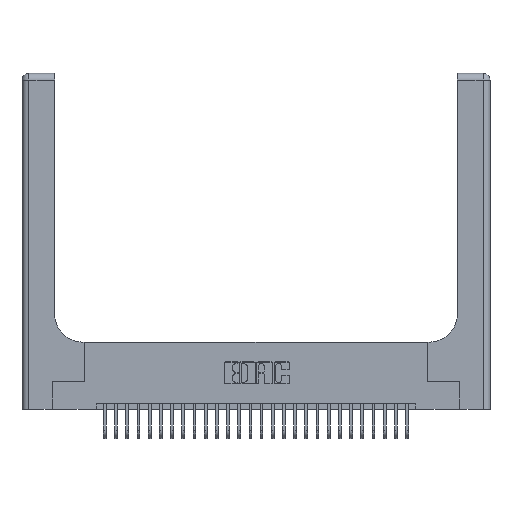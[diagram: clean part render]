
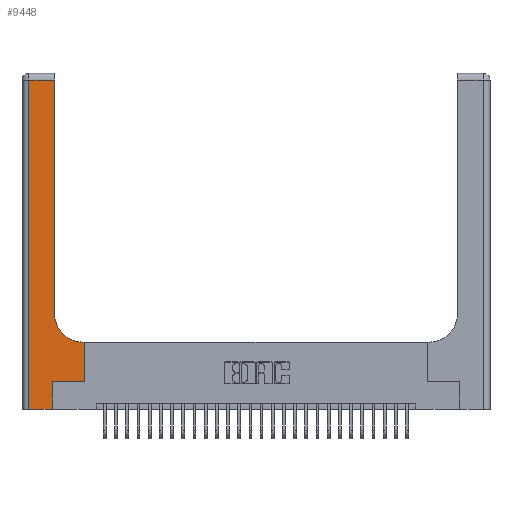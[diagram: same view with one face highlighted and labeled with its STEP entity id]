
A CAD part, top view. The second image highlights one B-rep face of the part: STEP entity #9448.
In plain terms, the highlighted planar face has unit normal (0, 0, 1).
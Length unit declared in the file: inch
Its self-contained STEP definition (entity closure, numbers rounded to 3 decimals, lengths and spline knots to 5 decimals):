
#297 = CARTESIAN_POINT ( 'NONE',  ( 0., 3., 0.37 ) ) ;
#1037 = CARTESIAN_POINT ( 'NONE',  ( 0.269, 0.25, 0.37 ) ) ;
#1071 = EDGE_CURVE ( 'NONE', #6506, #24500, #28959, .T. ) ;
#1226 = VECTOR ( 'NONE', #18215, 39.37008 ) ;
#2279 = ORIENTED_EDGE ( 'NONE', *, *, #6819, .T. ) ;
#3363 = DIRECTION ( 'NONE',  ( 0., -1., 0. ) ) ;
#3562 = EDGE_CURVE ( 'NONE', #7174, #15607, #13277, .T. ) ;
#3978 = EDGE_CURVE ( 'NONE', #15607, #24479, #28033, .T. ) ;
#5004 = PLANE ( 'NONE',  #11154 ) ;
#5107 = DIRECTION ( 'NONE',  ( -1., 0., 0. ) ) ;
#5175 = EDGE_CURVE ( 'NONE', #20872, #12508, #20188, .T. ) ;
#5329 = CARTESIAN_POINT ( 'NONE',  ( 0.5585, 0.6, 0.37 ) ) ;
#5599 = EDGE_CURVE ( 'NONE', #24479, #21643, #9063, .T. ) ;
#6296 = ORIENTED_EDGE ( 'NONE', *, *, #5175, .T. ) ;
#6438 = CARTESIAN_POINT ( 'NONE',  ( 0.06, 0., 0.37 ) ) ;
#6506 = VERTEX_POINT ( 'NONE', #30157 ) ;
#6819 = EDGE_CURVE ( 'NONE', #18335, #6506, #7108, .T. ) ;
#6947 = DIRECTION ( 'NONE',  ( 0., 1., 0. ) ) ;
#7108 = LINE ( 'NONE', #7600, #19004 ) ;
#7174 = VERTEX_POINT ( 'NONE', #6438 ) ;
#7600 = CARTESIAN_POINT ( 'NONE',  ( 0.2915, 0.6, 0.37 ) ) ;
#7916 = CARTESIAN_POINT ( 'NONE',  ( 0.2915, 0.85, 0.37 ) ) ;
#8496 = DIRECTION ( 'NONE',  ( 0., 0., -1. ) ) ;
#8878 = LINE ( 'NONE', #11604, #13674 ) ;
#8983 = LINE ( 'NONE', #17615, #21556 ) ;
#9063 = LINE ( 'NONE', #1037, #14609 ) ;
#9194 = VECTOR ( 'NONE', #16096, 39.37008 ) ;
#9448 = ADVANCED_FACE ( 'NONE', ( #24695 ), #5004, .F. ) ;
#10144 = DIRECTION ( 'NONE',  ( 0., 1., 0. ) ) ;
#10786 = ORIENTED_EDGE ( 'NONE', *, *, #28792, .T. ) ;
#11154 = AXIS2_PLACEMENT_3D ( 'NONE', #297, #19344, #5107 ) ;
#11604 = CARTESIAN_POINT ( 'NONE',  ( 0.2915, 3., 0.37 ) ) ;
#11655 = ORIENTED_EDGE ( 'NONE', *, *, #3978, .T. ) ;
#12508 = VERTEX_POINT ( 'NONE', #23676 ) ;
#12780 = EDGE_CURVE ( 'NONE', #12508, #7174, #8983, .T. ) ;
#13107 = ORIENTED_EDGE ( 'NONE', *, *, #3562, .T. ) ;
#13277 = LINE ( 'NONE', #28307, #19588 ) ;
#13674 = VECTOR ( 'NONE', #6947, 39.37008 ) ;
#13714 = CARTESIAN_POINT ( 'NONE',  ( 0.269, 0., 0.37 ) ) ;
#14431 = ORIENTED_EDGE ( 'NONE', *, *, #12780, .T. ) ;
#14609 = VECTOR ( 'NONE', #27053, 39.37008 ) ;
#14793 = AXIS2_PLACEMENT_3D ( 'NONE', #22649, #8496, #25015 ) ;
#15607 = VERTEX_POINT ( 'NONE', #27298 ) ;
#16096 = DIRECTION ( 'NONE',  ( 0., 1., 0. ) ) ;
#16605 = LINE ( 'NONE', #17167, #22137 ) ;
#17079 = ORIENTED_EDGE ( 'NONE', *, *, #1071, .T. ) ;
#17167 = CARTESIAN_POINT ( 'NONE',  ( 0.5585, 0.25, 0.37 ) ) ;
#17615 = CARTESIAN_POINT ( 'NONE',  ( 0.06, 3., 0.37 ) ) ;
#18215 = DIRECTION ( 'NONE',  ( -1., 0., 0. ) ) ;
#18334 = EDGE_CURVE ( 'NONE', #21643, #18335, #16605, .T. ) ;
#18335 = VERTEX_POINT ( 'NONE', #5329 ) ;
#19004 = VECTOR ( 'NONE', #28909, 39.37008 ) ;
#19344 = DIRECTION ( 'NONE',  ( 0., 0., -1. ) ) ;
#19588 = VECTOR ( 'NONE', #30686, 39.37008 ) ;
#19724 = CARTESIAN_POINT ( 'NONE',  ( 0.269, 0.25, 0.37 ) ) ;
#20188 = LINE ( 'NONE', #29944, #1226 ) ;
#20872 = VERTEX_POINT ( 'NONE', #29404 ) ;
#21476 = EDGE_LOOP ( 'NONE', ( #10786, #6296, #14431, #13107, #11655, #26760, #26188, #2279, #17079 ) ) ;
#21556 = VECTOR ( 'NONE', #3363, 39.37008 ) ;
#21643 = VERTEX_POINT ( 'NONE', #27486 ) ;
#22137 = VECTOR ( 'NONE', #10144, 39.37008 ) ;
#22649 = CARTESIAN_POINT ( 'NONE',  ( 0.5415, 0.85, 0.37 ) ) ;
#23676 = CARTESIAN_POINT ( 'NONE',  ( 0.06, 2.94, 0.37 ) ) ;
#24479 = VERTEX_POINT ( 'NONE', #19724 ) ;
#24500 = VERTEX_POINT ( 'NONE', #7916 ) ;
#24695 = FACE_OUTER_BOUND ( 'NONE', #21476, .T. ) ;
#25015 = DIRECTION ( 'NONE',  ( 1., 0., 0. ) ) ;
#26188 = ORIENTED_EDGE ( 'NONE', *, *, #18334, .T. ) ;
#26760 = ORIENTED_EDGE ( 'NONE', *, *, #5599, .T. ) ;
#27053 = DIRECTION ( 'NONE',  ( 1., 0., 0. ) ) ;
#27298 = CARTESIAN_POINT ( 'NONE',  ( 0.269, 0., 0.37 ) ) ;
#27486 = CARTESIAN_POINT ( 'NONE',  ( 0.5585, 0.25, 0.37 ) ) ;
#28033 = LINE ( 'NONE', #13714, #9194 ) ;
#28307 = CARTESIAN_POINT ( 'NONE',  ( 0., 0., 0.37 ) ) ;
#28792 = EDGE_CURVE ( 'NONE', #24500, #20872, #8878, .T. ) ;
#28909 = DIRECTION ( 'NONE',  ( -1., 0., 0. ) ) ;
#28959 = CIRCLE ( 'NONE', #14793, 0.25 ) ;
#29404 = CARTESIAN_POINT ( 'NONE',  ( 0.2915, 2.94, 0.37 ) ) ;
#29944 = CARTESIAN_POINT ( 'NONE',  ( 0., 2.94, 0.37 ) ) ;
#30157 = CARTESIAN_POINT ( 'NONE',  ( 0.5415, 0.6, 0.37 ) ) ;
#30686 = DIRECTION ( 'NONE',  ( 1., 0., 0. ) ) ;
